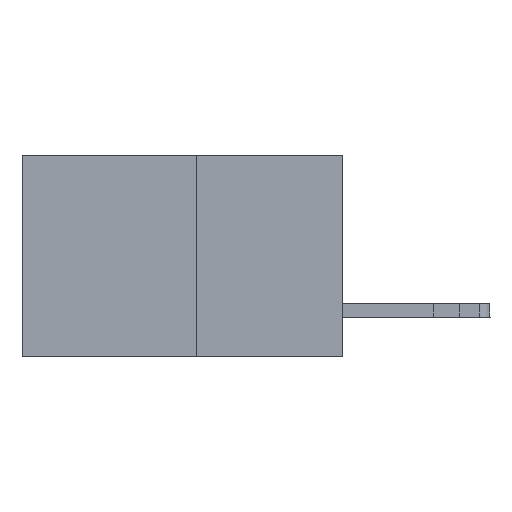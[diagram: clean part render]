
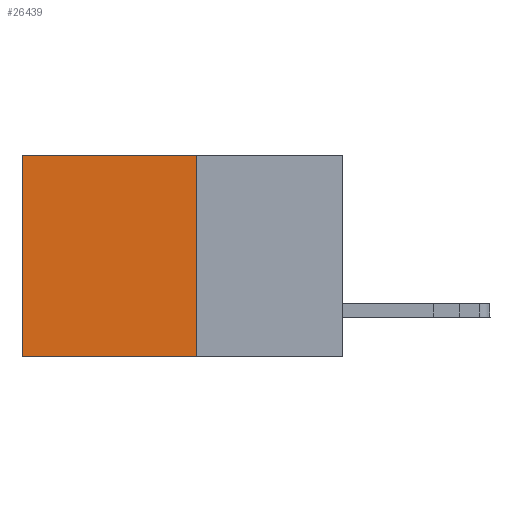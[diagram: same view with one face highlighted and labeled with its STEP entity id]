
A CAD part, left-side view. The second image highlights one B-rep face of the part: STEP entity #26439.
In plain terms, the highlighted planar face has unit normal (-1, 0, 0).
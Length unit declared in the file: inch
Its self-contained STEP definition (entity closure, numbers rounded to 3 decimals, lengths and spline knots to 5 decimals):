
#72 = DIRECTION ( 'NONE',  ( 0., 1., 0. ) ) ;
#742 = DIRECTION ( 'NONE',  ( 0., 0., -1. ) ) ;
#1065 = ORIENTED_EDGE ( 'NONE', *, *, #5604, .F. ) ;
#2866 = LINE ( 'NONE', #20166, #5165 ) ;
#3211 = VECTOR ( 'NONE', #72, 39.37008 ) ;
#4765 = ORIENTED_EDGE ( 'NONE', *, *, #5045, .T. ) ;
#4819 = CARTESIAN_POINT ( 'NONE',  ( 0.277, 0.27, 0. ) ) ;
#5040 = EDGE_LOOP ( 'NONE', ( #4765, #20626, #1065, #7655 ) ) ;
#5045 = EDGE_CURVE ( 'NONE', #21665, #23360, #2866, .T. ) ;
#5165 = VECTOR ( 'NONE', #742, 39.37008 ) ;
#5245 = CARTESIAN_POINT ( 'NONE',  ( 0.277, 0.27, -0.37 ) ) ;
#5363 = DIRECTION ( 'NONE',  ( 0., 1., 0. ) ) ;
#5423 = VERTEX_POINT ( 'NONE', #5245 ) ;
#5604 = EDGE_CURVE ( 'NONE', #15995, #5423, #16310, .T. ) ;
#7332 = DIRECTION ( 'NONE',  ( 1., 0., 0. ) ) ;
#7655 = ORIENTED_EDGE ( 'NONE', *, *, #12605, .T. ) ;
#9601 = DIRECTION ( 'NONE',  ( 0., 0., -1. ) ) ;
#9785 = AXIS2_PLACEMENT_3D ( 'NONE', #15997, #7332, #9601 ) ;
#10272 = EDGE_CURVE ( 'NONE', #5423, #23360, #25892, .T. ) ;
#10862 = CARTESIAN_POINT ( 'NONE',  ( 0.277, 0.27, -0.37 ) ) ;
#11455 = FACE_OUTER_BOUND ( 'NONE', #5040, .T. ) ;
#12605 = EDGE_CURVE ( 'NONE', #15995, #21665, #27340, .T. ) ;
#12610 = DIRECTION ( 'NONE',  ( 0., 0., -1. ) ) ;
#14154 = CARTESIAN_POINT ( 'NONE',  ( 0.277, 0.27, 0. ) ) ;
#14287 = VECTOR ( 'NONE', #12610, 39.37008 ) ;
#15995 = VERTEX_POINT ( 'NONE', #4819 ) ;
#15997 = CARTESIAN_POINT ( 'NONE',  ( 0.277, 0.27, -0.37 ) ) ;
#16310 = LINE ( 'NONE', #27523, #14287 ) ;
#18182 = CARTESIAN_POINT ( 'NONE',  ( 0.277, 0.59, 0. ) ) ;
#19627 = CARTESIAN_POINT ( 'NONE',  ( 0.277, 0.59, -0.37 ) ) ;
#20166 = CARTESIAN_POINT ( 'NONE',  ( 0.277, 0.59, -0.37 ) ) ;
#20626 = ORIENTED_EDGE ( 'NONE', *, *, #10272, .F. ) ;
#21665 = VERTEX_POINT ( 'NONE', #18182 ) ;
#21776 = VECTOR ( 'NONE', #5363, 39.37008 ) ;
#22519 = PLANE ( 'NONE',  #9785 ) ;
#23360 = VERTEX_POINT ( 'NONE', #19627 ) ;
#25892 = LINE ( 'NONE', #10862, #3211 ) ;
#26439 = ADVANCED_FACE ( 'NONE', ( #11455 ), #22519, .F. ) ;
#27340 = LINE ( 'NONE', #14154, #21776 ) ;
#27523 = CARTESIAN_POINT ( 'NONE',  ( 0.277, 0.27, -0.37 ) ) ;
